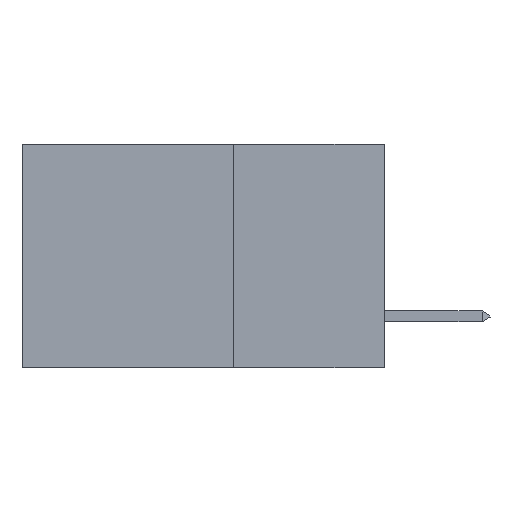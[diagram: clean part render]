
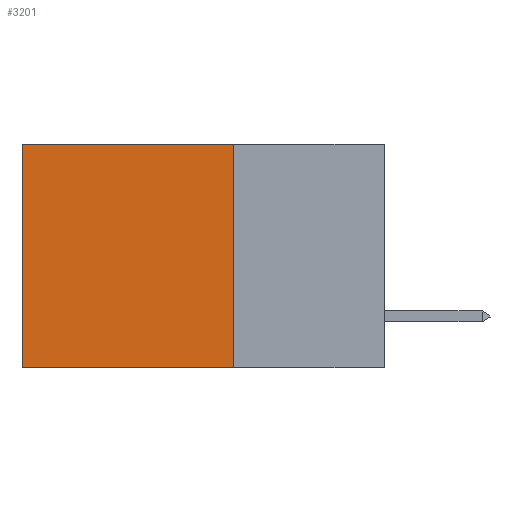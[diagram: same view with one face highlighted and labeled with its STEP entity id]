
A CAD part, left-side view. The second image highlights one B-rep face of the part: STEP entity #3201.
In plain terms, the highlighted planar face has unit normal (-1, 0, 0).
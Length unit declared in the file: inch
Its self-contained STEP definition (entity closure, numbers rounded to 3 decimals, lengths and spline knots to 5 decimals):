
#302 = LINE ( 'NONE', #3212, #10267 ) ;
#792 = CARTESIAN_POINT ( 'NONE',  ( 0.2875, 0.6, 0. ) ) ;
#1106 = EDGE_CURVE ( 'NONE', #16690, #1145, #18187, .T. ) ;
#1145 = VERTEX_POINT ( 'NONE', #9844 ) ;
#2448 = CARTESIAN_POINT ( 'NONE',  ( 0.2875, 0.25, 0. ) ) ;
#3201 = ADVANCED_FACE ( 'NONE', ( #15405 ), #12876, .F. ) ;
#3212 = CARTESIAN_POINT ( 'NONE',  ( 0.2875, 0.25, 0. ) ) ;
#3213 = CARTESIAN_POINT ( 'NONE',  ( 0.2875, 0.25, 0. ) ) ;
#3535 = EDGE_CURVE ( 'NONE', #11529, #1145, #14488, .T. ) ;
#4324 = CARTESIAN_POINT ( 'NONE',  ( 0.2875, 0.25, 0. ) ) ;
#4738 = VECTOR ( 'NONE', #12665, 39.37008 ) ;
#5248 = ORIENTED_EDGE ( 'NONE', *, *, #8573, .F. ) ;
#5918 = VECTOR ( 'NONE', #15300, 39.37008 ) ;
#6196 = EDGE_CURVE ( 'NONE', #16351, #16690, #302, .T. ) ;
#6538 = DIRECTION ( 'NONE',  ( 0., 0., -1. ) ) ;
#8458 = AXIS2_PLACEMENT_3D ( 'NONE', #4324, #11415, #11480 ) ;
#8573 = EDGE_CURVE ( 'NONE', #16351, #11529, #12951, .T. ) ;
#8622 = ORIENTED_EDGE ( 'NONE', *, *, #1106, .T. ) ;
#8712 = DIRECTION ( 'NONE',  ( 0., 1., 0. ) ) ;
#9844 = CARTESIAN_POINT ( 'NONE',  ( 0.2875, 0.6, -0.37 ) ) ;
#10201 = ORIENTED_EDGE ( 'NONE', *, *, #3535, .F. ) ;
#10267 = VECTOR ( 'NONE', #8712, 39.37008 ) ;
#11025 = CARTESIAN_POINT ( 'NONE',  ( 0.2875, 0.25, -0.37 ) ) ;
#11415 = DIRECTION ( 'NONE',  ( 1., 0., 0. ) ) ;
#11480 = DIRECTION ( 'NONE',  ( 0., 0., -1. ) ) ;
#11529 = VERTEX_POINT ( 'NONE', #16696 ) ;
#11853 = VECTOR ( 'NONE', #6538, 39.37008 ) ;
#11962 = EDGE_LOOP ( 'NONE', ( #8622, #10201, #5248, #16290 ) ) ;
#12665 = DIRECTION ( 'NONE',  ( 0., 1., 0. ) ) ;
#12876 = PLANE ( 'NONE',  #8458 ) ;
#12951 = LINE ( 'NONE', #2448, #5918 ) ;
#14488 = LINE ( 'NONE', #11025, #4738 ) ;
#15300 = DIRECTION ( 'NONE',  ( 0., 0., -1. ) ) ;
#15405 = FACE_OUTER_BOUND ( 'NONE', #11962, .T. ) ;
#16290 = ORIENTED_EDGE ( 'NONE', *, *, #6196, .T. ) ;
#16351 = VERTEX_POINT ( 'NONE', #3213 ) ;
#16690 = VERTEX_POINT ( 'NONE', #792 ) ;
#16696 = CARTESIAN_POINT ( 'NONE',  ( 0.2875, 0.25, -0.37 ) ) ;
#17953 = CARTESIAN_POINT ( 'NONE',  ( 0.2875, 0.6, 0. ) ) ;
#18187 = LINE ( 'NONE', #17953, #11853 ) ;
